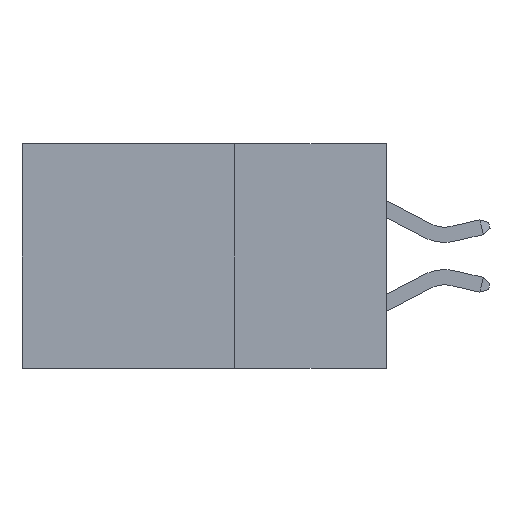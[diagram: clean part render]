
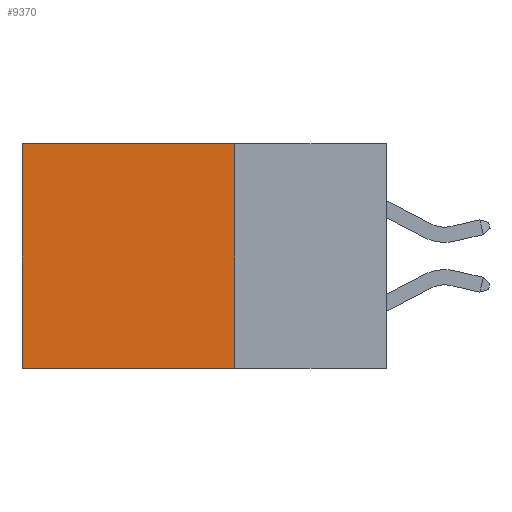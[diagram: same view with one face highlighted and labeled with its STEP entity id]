
A CAD part, left-side view. The second image highlights one B-rep face of the part: STEP entity #9370.
In plain terms, the highlighted planar face has unit normal (-1, 0, 0).
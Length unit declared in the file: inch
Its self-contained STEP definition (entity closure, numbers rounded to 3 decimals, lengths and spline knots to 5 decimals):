
#829 = ORIENTED_EDGE ( 'NONE', *, *, #15074, .F. ) ;
#2481 = CARTESIAN_POINT ( 'NONE',  ( 0.2615, 0.6, -0.37 ) ) ;
#2949 = EDGE_CURVE ( 'NONE', #17709, #9000, #17779, .T. ) ;
#3635 = CARTESIAN_POINT ( 'NONE',  ( 0.2615, 0.25, -0.37 ) ) ;
#4234 = DIRECTION ( 'NONE',  ( 0., 0., -1. ) ) ;
#4302 = VECTOR ( 'NONE', #4234, 39.37008 ) ;
#4505 = CARTESIAN_POINT ( 'NONE',  ( 0.2615, 0.25, -0.37 ) ) ;
#4947 = CARTESIAN_POINT ( 'NONE',  ( 0.2615, 0.25, -0.37 ) ) ;
#5058 = DIRECTION ( 'NONE',  ( 1., 0., 0. ) ) ;
#6707 = CARTESIAN_POINT ( 'NONE',  ( 0.2615, 0.6, 0. ) ) ;
#7685 = CARTESIAN_POINT ( 'NONE',  ( 0.2615, 0.25, -0.37 ) ) ;
#8021 = VECTOR ( 'NONE', #11179, 39.37008 ) ;
#8322 = DIRECTION ( 'NONE',  ( 0., 0., -1. ) ) ;
#8751 = CARTESIAN_POINT ( 'NONE',  ( 0.2615, 0.25, 0. ) ) ;
#8963 = DIRECTION ( 'NONE',  ( 0., 1., 0. ) ) ;
#9000 = VERTEX_POINT ( 'NONE', #13219 ) ;
#9163 = VERTEX_POINT ( 'NONE', #7685 ) ;
#9370 = ADVANCED_FACE ( 'NONE', ( #13233 ), #18282, .F. ) ;
#9383 = EDGE_CURVE ( 'NONE', #10339, #9163, #13450, .T. ) ;
#10339 = VERTEX_POINT ( 'NONE', #12319 ) ;
#10676 = ORIENTED_EDGE ( 'NONE', *, *, #13135, .T. ) ;
#11003 = VECTOR ( 'NONE', #8322, 39.37008 ) ;
#11179 = DIRECTION ( 'NONE',  ( 0., 1., 0. ) ) ;
#12319 = CARTESIAN_POINT ( 'NONE',  ( 0.2615, 0.25, 0. ) ) ;
#12915 = LINE ( 'NONE', #4505, #8021 ) ;
#13135 = EDGE_CURVE ( 'NONE', #10339, #17709, #13434, .T. ) ;
#13219 = CARTESIAN_POINT ( 'NONE',  ( 0.2615, 0.6, -0.37 ) ) ;
#13233 = FACE_OUTER_BOUND ( 'NONE', #21406, .T. ) ;
#13434 = LINE ( 'NONE', #8751, #17007 ) ;
#13450 = LINE ( 'NONE', #4947, #11003 ) ;
#15074 = EDGE_CURVE ( 'NONE', #9163, #9000, #12915, .T. ) ;
#16956 = AXIS2_PLACEMENT_3D ( 'NONE', #3635, #5058, #19921 ) ;
#17007 = VECTOR ( 'NONE', #8963, 39.37008 ) ;
#17709 = VERTEX_POINT ( 'NONE', #6707 ) ;
#17779 = LINE ( 'NONE', #2481, #4302 ) ;
#17982 = ORIENTED_EDGE ( 'NONE', *, *, #2949, .T. ) ;
#18030 = ORIENTED_EDGE ( 'NONE', *, *, #9383, .F. ) ;
#18282 = PLANE ( 'NONE',  #16956 ) ;
#19921 = DIRECTION ( 'NONE',  ( 0., 0., -1. ) ) ;
#21406 = EDGE_LOOP ( 'NONE', ( #17982, #829, #18030, #10676 ) ) ;
